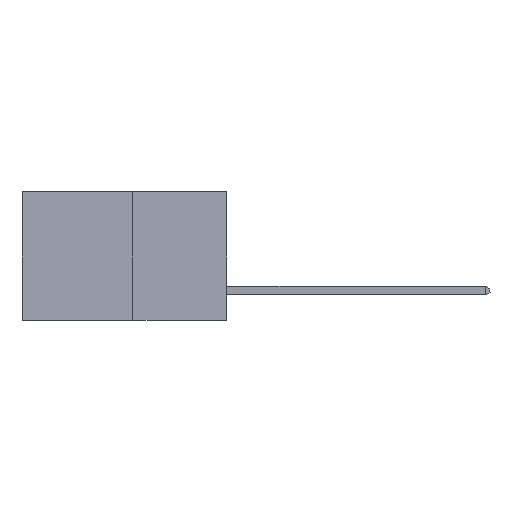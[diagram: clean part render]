
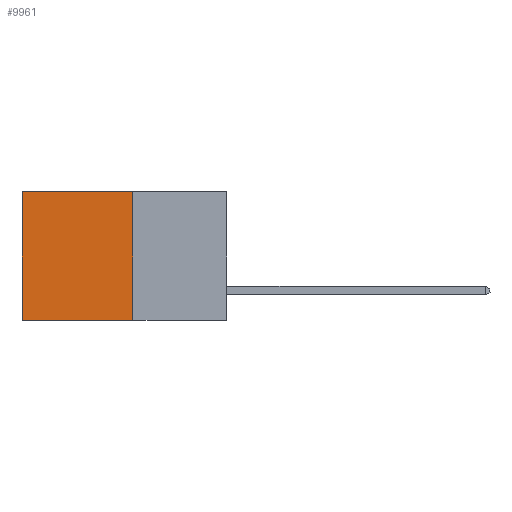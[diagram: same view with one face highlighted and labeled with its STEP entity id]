
A CAD part, left-side view. The second image highlights one B-rep face of the part: STEP entity #9961.
In plain terms, the highlighted planar face has unit normal (-1, 0, 0).
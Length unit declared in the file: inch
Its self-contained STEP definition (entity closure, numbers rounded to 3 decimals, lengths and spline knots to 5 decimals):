
#354 = CARTESIAN_POINT ( 'NONE',  ( 0.277, 0.59, 0. ) ) ;
#366 = VECTOR ( 'NONE', #8969, 39.37008 ) ;
#561 = FACE_OUTER_BOUND ( 'NONE', #1497, .T. ) ;
#601 = VERTEX_POINT ( 'NONE', #2434 ) ;
#690 = VERTEX_POINT ( 'NONE', #354 ) ;
#857 = EDGE_CURVE ( 'NONE', #1844, #690, #5221, .T. ) ;
#1114 = ORIENTED_EDGE ( 'NONE', *, *, #9040, .F. ) ;
#1353 = ORIENTED_EDGE ( 'NONE', *, *, #857, .T. ) ;
#1497 = EDGE_LOOP ( 'NONE', ( #9261, #6359, #1114, #1353 ) ) ;
#1844 = VERTEX_POINT ( 'NONE', #2314 ) ;
#1874 = DIRECTION ( 'NONE',  ( 1., 0., 0. ) ) ;
#2314 = CARTESIAN_POINT ( 'NONE',  ( 0.277, 0.27, 0. ) ) ;
#2434 = CARTESIAN_POINT ( 'NONE',  ( 0.277, 0.27, -0.37 ) ) ;
#2871 = EDGE_CURVE ( 'NONE', #690, #9213, #7349, .T. ) ;
#3667 = DIRECTION ( 'NONE',  ( 0., 1., 0. ) ) ;
#4404 = CARTESIAN_POINT ( 'NONE',  ( 0.277, 0.59, -0.37 ) ) ;
#4407 = DIRECTION ( 'NONE',  ( 0., 0., -1. ) ) ;
#5221 = LINE ( 'NONE', #8929, #366 ) ;
#6359 = ORIENTED_EDGE ( 'NONE', *, *, #6795, .F. ) ;
#6795 = EDGE_CURVE ( 'NONE', #601, #9213, #11650, .T. ) ;
#7063 = VECTOR ( 'NONE', #4407, 39.37008 ) ;
#7165 = LINE ( 'NONE', #7614, #11855 ) ;
#7349 = LINE ( 'NONE', #4404, #7063 ) ;
#7585 = CARTESIAN_POINT ( 'NONE',  ( 0.277, 0.27, -0.37 ) ) ;
#7614 = CARTESIAN_POINT ( 'NONE',  ( 0.277, 0.27, -0.37 ) ) ;
#8481 = DIRECTION ( 'NONE',  ( 0., 0., -1. ) ) ;
#8929 = CARTESIAN_POINT ( 'NONE',  ( 0.277, 0.27, 0. ) ) ;
#8969 = DIRECTION ( 'NONE',  ( 0., 1., 0. ) ) ;
#9040 = EDGE_CURVE ( 'NONE', #1844, #601, #7165, .T. ) ;
#9200 = CARTESIAN_POINT ( 'NONE',  ( 0.277, 0.27, -0.37 ) ) ;
#9213 = VERTEX_POINT ( 'NONE', #11127 ) ;
#9261 = ORIENTED_EDGE ( 'NONE', *, *, #2871, .T. ) ;
#9395 = DIRECTION ( 'NONE',  ( 0., 0., -1. ) ) ;
#9961 = ADVANCED_FACE ( 'NONE', ( #561 ), #11951, .F. ) ;
#10938 = AXIS2_PLACEMENT_3D ( 'NONE', #7585, #1874, #8481 ) ;
#11127 = CARTESIAN_POINT ( 'NONE',  ( 0.277, 0.59, -0.37 ) ) ;
#11650 = LINE ( 'NONE', #9200, #11912 ) ;
#11855 = VECTOR ( 'NONE', #9395, 39.37008 ) ;
#11912 = VECTOR ( 'NONE', #3667, 39.37008 ) ;
#11951 = PLANE ( 'NONE',  #10938 ) ;
